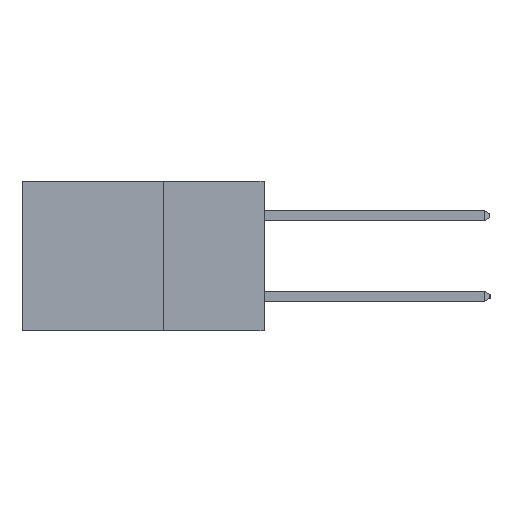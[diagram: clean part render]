
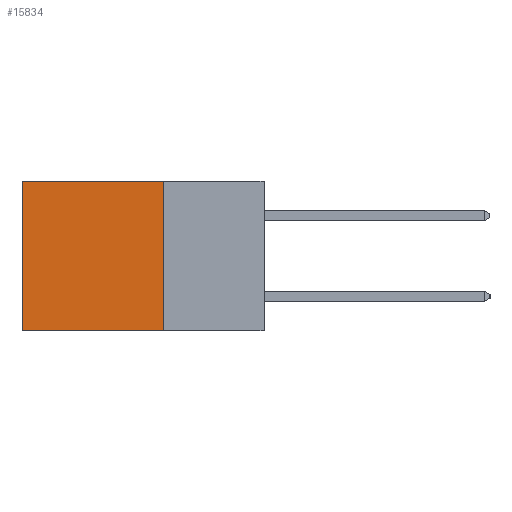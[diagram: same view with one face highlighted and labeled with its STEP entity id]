
A CAD part, left-side view. The second image highlights one B-rep face of the part: STEP entity #15834.
In plain terms, the highlighted planar face has unit normal (-1, 0, 0).
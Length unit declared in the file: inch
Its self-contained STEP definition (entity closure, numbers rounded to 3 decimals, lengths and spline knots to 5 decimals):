
#412 = CARTESIAN_POINT ( 'NONE',  ( 0.2615, 0.25, 0. ) ) ;
#899 = CARTESIAN_POINT ( 'NONE',  ( 0.2615, 0.25, -0.37 ) ) ;
#1232 = LINE ( 'NONE', #899, #5127 ) ;
#2216 = VERTEX_POINT ( 'NONE', #18025 ) ;
#2344 = DIRECTION ( 'NONE',  ( 0., 1., 0. ) ) ;
#3348 = DIRECTION ( 'NONE',  ( 0., 1., 0. ) ) ;
#3659 = DIRECTION ( 'NONE',  ( 1., 0., 0. ) ) ;
#4009 = CARTESIAN_POINT ( 'NONE',  ( 0.2615, 0.6, -0.37 ) ) ;
#4201 = LINE ( 'NONE', #13112, #5845 ) ;
#4469 = EDGE_LOOP ( 'NONE', ( #18569, #11402, #12758, #12668 ) ) ;
#5127 = VECTOR ( 'NONE', #2344, 39.37008 ) ;
#5378 = EDGE_CURVE ( 'NONE', #2216, #16700, #4201, .T. ) ;
#5845 = VECTOR ( 'NONE', #12918, 39.37008 ) ;
#6806 = AXIS2_PLACEMENT_3D ( 'NONE', #12511, #3659, #13985 ) ;
#6840 = VERTEX_POINT ( 'NONE', #13444 ) ;
#7047 = CARTESIAN_POINT ( 'NONE',  ( 0.2615, 0.25, -0.37 ) ) ;
#7928 = VERTEX_POINT ( 'NONE', #7047 ) ;
#8687 = VECTOR ( 'NONE', #3348, 39.37008 ) ;
#9163 = LINE ( 'NONE', #412, #8687 ) ;
#9557 = PLANE ( 'NONE',  #6806 ) ;
#10216 = EDGE_CURVE ( 'NONE', #6840, #2216, #9163, .T. ) ;
#10489 = VECTOR ( 'NONE', #14707, 39.37008 ) ;
#11385 = EDGE_CURVE ( 'NONE', #6840, #7928, #18268, .T. ) ;
#11402 = ORIENTED_EDGE ( 'NONE', *, *, #13006, .F. ) ;
#12511 = CARTESIAN_POINT ( 'NONE',  ( 0.2615, 0.25, -0.37 ) ) ;
#12668 = ORIENTED_EDGE ( 'NONE', *, *, #10216, .T. ) ;
#12758 = ORIENTED_EDGE ( 'NONE', *, *, #11385, .F. ) ;
#12918 = DIRECTION ( 'NONE',  ( 0., 0., -1. ) ) ;
#13006 = EDGE_CURVE ( 'NONE', #7928, #16700, #1232, .T. ) ;
#13112 = CARTESIAN_POINT ( 'NONE',  ( 0.2615, 0.6, -0.37 ) ) ;
#13242 = CARTESIAN_POINT ( 'NONE',  ( 0.2615, 0.25, -0.37 ) ) ;
#13444 = CARTESIAN_POINT ( 'NONE',  ( 0.2615, 0.25, 0. ) ) ;
#13985 = DIRECTION ( 'NONE',  ( 0., 0., -1. ) ) ;
#14707 = DIRECTION ( 'NONE',  ( 0., 0., -1. ) ) ;
#15834 = ADVANCED_FACE ( 'NONE', ( #17700 ), #9557, .F. ) ;
#16700 = VERTEX_POINT ( 'NONE', #4009 ) ;
#17700 = FACE_OUTER_BOUND ( 'NONE', #4469, .T. ) ;
#18025 = CARTESIAN_POINT ( 'NONE',  ( 0.2615, 0.6, 0. ) ) ;
#18268 = LINE ( 'NONE', #13242, #10489 ) ;
#18569 = ORIENTED_EDGE ( 'NONE', *, *, #5378, .T. ) ;
